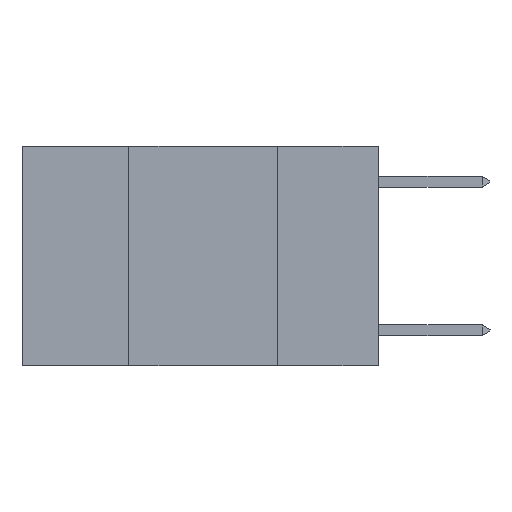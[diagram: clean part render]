
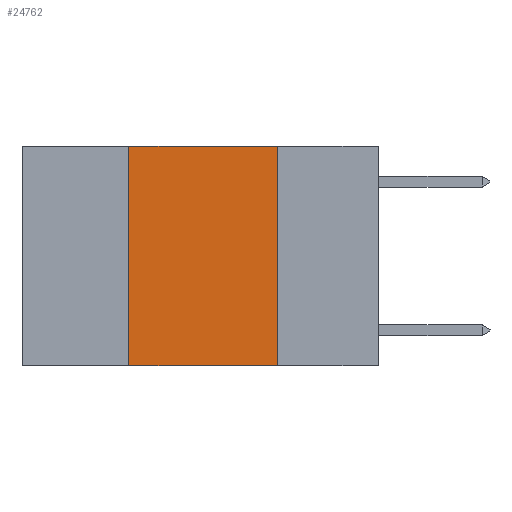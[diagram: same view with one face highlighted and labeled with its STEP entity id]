
A CAD part, left-side view. The second image highlights one B-rep face of the part: STEP entity #24762.
In plain terms, the highlighted planar face has unit normal (-1, 0, 0).
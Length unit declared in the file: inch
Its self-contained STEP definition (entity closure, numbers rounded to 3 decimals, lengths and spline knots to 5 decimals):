
#239 = EDGE_CURVE ( 'NONE', #23533, #11175, #25261, .T. ) ;
#258 = DIRECTION ( 'NONE',  ( 0., -1., 0. ) ) ;
#1435 = CARTESIAN_POINT ( 'NONE',  ( 0., 0.6, -0.37 ) ) ;
#1522 = ORIENTED_EDGE ( 'NONE', *, *, #2070, .F. ) ;
#1823 = ORIENTED_EDGE ( 'NONE', *, *, #16220, .F. ) ;
#2070 = EDGE_CURVE ( 'NONE', #9032, #11175, #15510, .T. ) ;
#2392 = VECTOR ( 'NONE', #23185, 39.37008 ) ;
#4086 = ORIENTED_EDGE ( 'NONE', *, *, #4403, .F. ) ;
#4403 = EDGE_CURVE ( 'NONE', #23533, #16665, #29087, .T. ) ;
#7218 = ORIENTED_EDGE ( 'NONE', *, *, #239, .T. ) ;
#8798 = AXIS2_PLACEMENT_3D ( 'NONE', #28985, #31289, #17001 ) ;
#9032 = VERTEX_POINT ( 'NONE', #21429 ) ;
#10370 = DIRECTION ( 'NONE',  ( 0., -1., 0. ) ) ;
#11175 = VERTEX_POINT ( 'NONE', #21818 ) ;
#12117 = PLANE ( 'NONE',  #8798 ) ;
#14259 = DIRECTION ( 'NONE',  ( 0., 0., -1. ) ) ;
#14938 = VECTOR ( 'NONE', #14259, 39.37008 ) ;
#15510 = LINE ( 'NONE', #21470, #14938 ) ;
#16220 = EDGE_CURVE ( 'NONE', #16665, #9032, #22321, .T. ) ;
#16665 = VERTEX_POINT ( 'NONE', #31097 ) ;
#16718 = VECTOR ( 'NONE', #10370, 39.37008 ) ;
#16960 = CARTESIAN_POINT ( 'NONE',  ( 0., 0.42, -0.37 ) ) ;
#16983 = EDGE_LOOP ( 'NONE', ( #1522, #1823, #4086, #7218 ) ) ;
#17001 = DIRECTION ( 'NONE',  ( 0., 0., -1. ) ) ;
#20782 = CARTESIAN_POINT ( 'NONE',  ( 0., 0.42, 0. ) ) ;
#21429 = CARTESIAN_POINT ( 'NONE',  ( 0., 0.17, 0. ) ) ;
#21470 = CARTESIAN_POINT ( 'NONE',  ( 0., 0.17, 0. ) ) ;
#21818 = CARTESIAN_POINT ( 'NONE',  ( 0., 0.17, -0.37 ) ) ;
#22089 = VECTOR ( 'NONE', #258, 39.37008 ) ;
#22321 = LINE ( 'NONE', #24815, #16718 ) ;
#23185 = DIRECTION ( 'NONE',  ( 0., 0., 1. ) ) ;
#23533 = VERTEX_POINT ( 'NONE', #16960 ) ;
#24274 = FACE_OUTER_BOUND ( 'NONE', #16983, .T. ) ;
#24762 = ADVANCED_FACE ( 'NONE', ( #24274 ), #12117, .F. ) ;
#24815 = CARTESIAN_POINT ( 'NONE',  ( 0., 0.6, 0. ) ) ;
#25261 = LINE ( 'NONE', #1435, #22089 ) ;
#28985 = CARTESIAN_POINT ( 'NONE',  ( 0., 0.6, 0. ) ) ;
#29087 = LINE ( 'NONE', #20782, #2392 ) ;
#31097 = CARTESIAN_POINT ( 'NONE',  ( 0., 0.42, 0. ) ) ;
#31289 = DIRECTION ( 'NONE',  ( 1., 0., 0. ) ) ;
